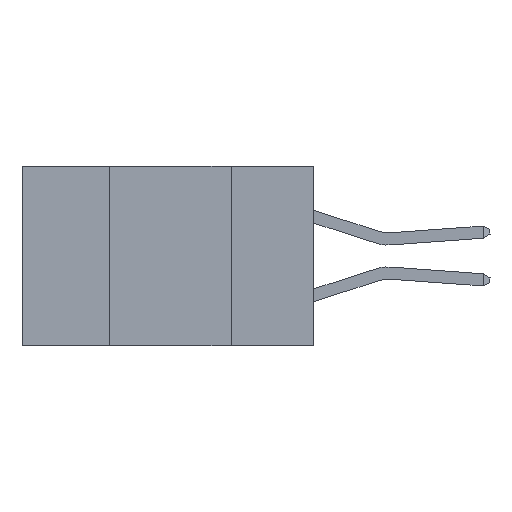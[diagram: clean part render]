
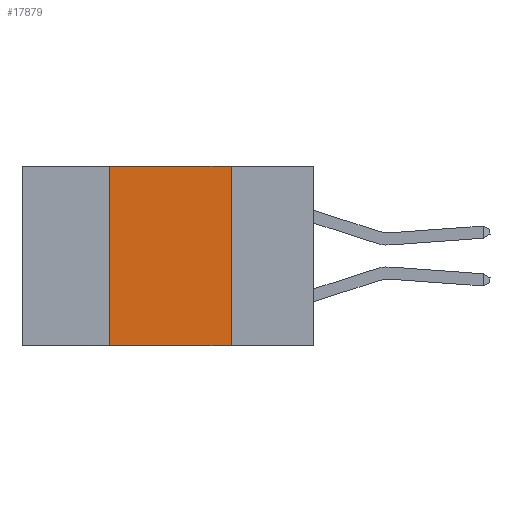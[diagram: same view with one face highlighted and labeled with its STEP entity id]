
A CAD part, left-side view. The second image highlights one B-rep face of the part: STEP entity #17879.
In plain terms, the highlighted planar face has unit normal (-1, 0, 0).
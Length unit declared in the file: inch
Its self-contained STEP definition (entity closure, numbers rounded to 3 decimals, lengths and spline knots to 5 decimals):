
#126 = CARTESIAN_POINT ( 'NONE',  ( 0., 0.17, 0. ) ) ;
#340 = DIRECTION ( 'NONE',  ( 0., -1., 0. ) ) ;
#814 = EDGE_CURVE ( 'NONE', #30340, #9280, #5061, .T. ) ;
#2566 = VECTOR ( 'NONE', #340, 39.37008 ) ;
#3492 = DIRECTION ( 'NONE',  ( 0., 0., 1. ) ) ;
#3758 = CARTESIAN_POINT ( 'NONE',  ( 0., 0.6, 0. ) ) ;
#4414 = CARTESIAN_POINT ( 'NONE',  ( 0., 0.42, 0. ) ) ;
#4678 = VECTOR ( 'NONE', #14829, 39.37008 ) ;
#5061 = LINE ( 'NONE', #17456, #4678 ) ;
#5844 = LINE ( 'NONE', #3758, #27202 ) ;
#6573 = VECTOR ( 'NONE', #3492, 39.37008 ) ;
#7247 = ORIENTED_EDGE ( 'NONE', *, *, #814, .F. ) ;
#8293 = DIRECTION ( 'NONE',  ( 1., 0., 0. ) ) ;
#9280 = VERTEX_POINT ( 'NONE', #23085 ) ;
#10735 = LINE ( 'NONE', #14558, #2566 ) ;
#11069 = VERTEX_POINT ( 'NONE', #4414 ) ;
#12055 = EDGE_CURVE ( 'NONE', #18950, #9280, #10735, .T. ) ;
#13063 = CARTESIAN_POINT ( 'NONE',  ( 0., 0.42, 0. ) ) ;
#14558 = CARTESIAN_POINT ( 'NONE',  ( 0., 0.6, -0.37 ) ) ;
#14691 = LINE ( 'NONE', #13063, #6573 ) ;
#14829 = DIRECTION ( 'NONE',  ( 0., 0., -1. ) ) ;
#15977 = DIRECTION ( 'NONE',  ( 0., -1., 0. ) ) ;
#17456 = CARTESIAN_POINT ( 'NONE',  ( 0., 0.17, 0. ) ) ;
#17879 = ADVANCED_FACE ( 'NONE', ( #25941 ), #27378, .F. ) ;
#18950 = VERTEX_POINT ( 'NONE', #28983 ) ;
#22193 = ORIENTED_EDGE ( 'NONE', *, *, #29345, .F. ) ;
#22463 = CARTESIAN_POINT ( 'NONE',  ( 0., 0.6, 0. ) ) ;
#23085 = CARTESIAN_POINT ( 'NONE',  ( 0., 0.17, -0.37 ) ) ;
#23094 = AXIS2_PLACEMENT_3D ( 'NONE', #22463, #8293, #27174 ) ;
#23434 = EDGE_CURVE ( 'NONE', #11069, #30340, #5844, .T. ) ;
#25941 = FACE_OUTER_BOUND ( 'NONE', #30562, .T. ) ;
#26718 = ORIENTED_EDGE ( 'NONE', *, *, #12055, .T. ) ;
#27174 = DIRECTION ( 'NONE',  ( 0., 0., -1. ) ) ;
#27202 = VECTOR ( 'NONE', #15977, 39.37008 ) ;
#27378 = PLANE ( 'NONE',  #23094 ) ;
#27771 = ORIENTED_EDGE ( 'NONE', *, *, #23434, .F. ) ;
#28983 = CARTESIAN_POINT ( 'NONE',  ( 0., 0.42, -0.37 ) ) ;
#29345 = EDGE_CURVE ( 'NONE', #18950, #11069, #14691, .T. ) ;
#30340 = VERTEX_POINT ( 'NONE', #126 ) ;
#30562 = EDGE_LOOP ( 'NONE', ( #7247, #27771, #22193, #26718 ) ) ;
